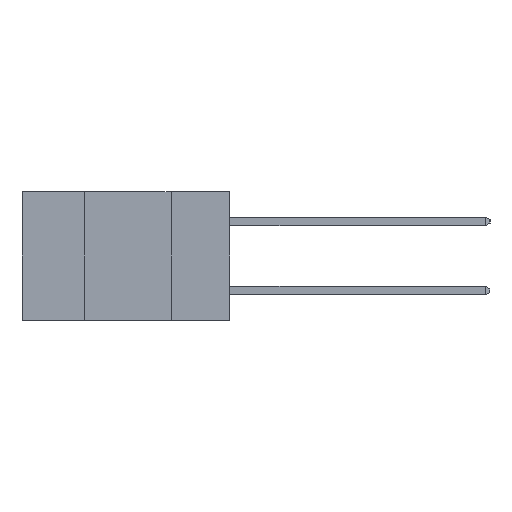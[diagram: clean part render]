
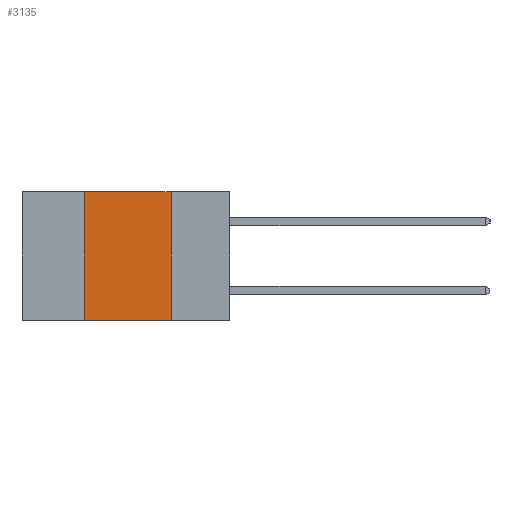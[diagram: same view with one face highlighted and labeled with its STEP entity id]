
A CAD part, left-side view. The second image highlights one B-rep face of the part: STEP entity #3135.
In plain terms, the highlighted planar face has unit normal (-1, 0, 0).
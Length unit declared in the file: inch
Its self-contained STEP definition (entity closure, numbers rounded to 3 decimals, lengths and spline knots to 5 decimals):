
#12 = EDGE_CURVE ( 'NONE', #1659, #12566, #4104, .T. ) ;
#282 = CARTESIAN_POINT ( 'NONE',  ( 0., 0.6, 0. ) ) ;
#935 = LINE ( 'NONE', #5659, #6515 ) ;
#1070 = VECTOR ( 'NONE', #4879, 39.37008 ) ;
#1659 = VERTEX_POINT ( 'NONE', #10523 ) ;
#2837 = EDGE_LOOP ( 'NONE', ( #5927, #7170, #12274, #12061 ) ) ;
#3038 = CARTESIAN_POINT ( 'NONE',  ( 0., 0.42, 0. ) ) ;
#3135 = ADVANCED_FACE ( 'NONE', ( #7258 ), #3497, .F. ) ;
#3394 = DIRECTION ( 'NONE',  ( 0., 0., -1. ) ) ;
#3438 = DIRECTION ( 'NONE',  ( 1., 0., 0. ) ) ;
#3497 = PLANE ( 'NONE',  #9578 ) ;
#3955 = CARTESIAN_POINT ( 'NONE',  ( 0., 0.6, 0. ) ) ;
#4104 = LINE ( 'NONE', #5892, #1070 ) ;
#4708 = DIRECTION ( 'NONE',  ( 0., 0., 1. ) ) ;
#4834 = DIRECTION ( 'NONE',  ( 0., -1., 0. ) ) ;
#4879 = DIRECTION ( 'NONE',  ( 0., -1., 0. ) ) ;
#5286 = VERTEX_POINT ( 'NONE', #11147 ) ;
#5659 = CARTESIAN_POINT ( 'NONE',  ( 0., 0.17, 0. ) ) ;
#5856 = EDGE_CURVE ( 'NONE', #1659, #9011, #7986, .T. ) ;
#5892 = CARTESIAN_POINT ( 'NONE',  ( 0., 0.6, -0.37 ) ) ;
#5927 = ORIENTED_EDGE ( 'NONE', *, *, #10754, .F. ) ;
#6515 = VECTOR ( 'NONE', #7873, 39.37008 ) ;
#6673 = VECTOR ( 'NONE', #4834, 39.37008 ) ;
#7139 = CARTESIAN_POINT ( 'NONE',  ( 0., 0.17, -0.37 ) ) ;
#7170 = ORIENTED_EDGE ( 'NONE', *, *, #10962, .F. ) ;
#7258 = FACE_OUTER_BOUND ( 'NONE', #2837, .T. ) ;
#7873 = DIRECTION ( 'NONE',  ( 0., 0., -1. ) ) ;
#7986 = LINE ( 'NONE', #12951, #13005 ) ;
#9011 = VERTEX_POINT ( 'NONE', #3038 ) ;
#9500 = LINE ( 'NONE', #282, #6673 ) ;
#9578 = AXIS2_PLACEMENT_3D ( 'NONE', #3955, #3438, #3394 ) ;
#10523 = CARTESIAN_POINT ( 'NONE',  ( 0., 0.42, -0.37 ) ) ;
#10754 = EDGE_CURVE ( 'NONE', #5286, #12566, #935, .T. ) ;
#10962 = EDGE_CURVE ( 'NONE', #9011, #5286, #9500, .T. ) ;
#11147 = CARTESIAN_POINT ( 'NONE',  ( 0., 0.17, 0. ) ) ;
#12061 = ORIENTED_EDGE ( 'NONE', *, *, #12, .T. ) ;
#12274 = ORIENTED_EDGE ( 'NONE', *, *, #5856, .F. ) ;
#12566 = VERTEX_POINT ( 'NONE', #7139 ) ;
#12951 = CARTESIAN_POINT ( 'NONE',  ( 0., 0.42, 0. ) ) ;
#13005 = VECTOR ( 'NONE', #4708, 39.37008 ) ;
